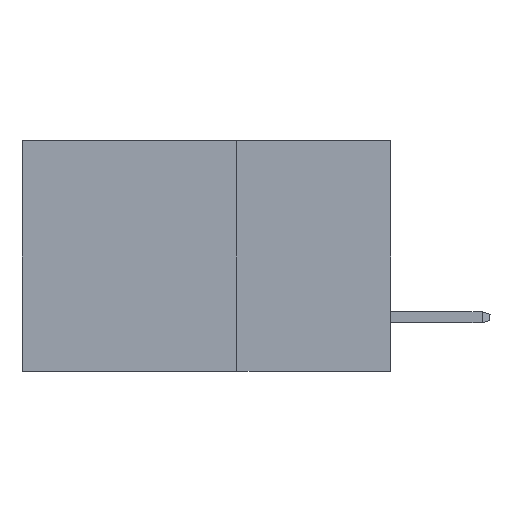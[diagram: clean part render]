
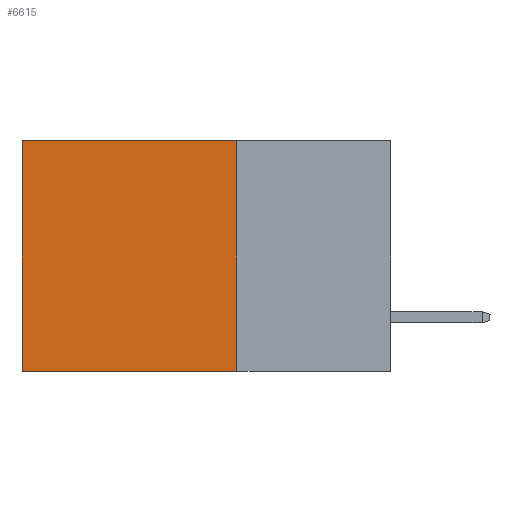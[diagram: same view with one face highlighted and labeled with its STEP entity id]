
A CAD part, left-side view. The second image highlights one B-rep face of the part: STEP entity #6615.
In plain terms, the highlighted planar face has unit normal (-1, 0, 0).
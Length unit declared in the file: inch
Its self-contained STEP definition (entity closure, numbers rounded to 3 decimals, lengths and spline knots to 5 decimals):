
#156 = CARTESIAN_POINT ( 'NONE',  ( 0.2875, 0.25, 0. ) ) ;
#399 = LINE ( 'NONE', #2664, #13032 ) ;
#751 = VERTEX_POINT ( 'NONE', #4200 ) ;
#1082 = LINE ( 'NONE', #13899, #9102 ) ;
#1190 = ORIENTED_EDGE ( 'NONE', *, *, #13895, .F. ) ;
#1422 = EDGE_LOOP ( 'NONE', ( #9313, #1190, #11334, #9749 ) ) ;
#2226 = DIRECTION ( 'NONE',  ( 0., 1., 0. ) ) ;
#2263 = VERTEX_POINT ( 'NONE', #10143 ) ;
#2664 = CARTESIAN_POINT ( 'NONE',  ( 0.2875, 0.25, 0. ) ) ;
#2682 = VECTOR ( 'NONE', #8875, 39.37008 ) ;
#2790 = AXIS2_PLACEMENT_3D ( 'NONE', #8000, #9123, #12720 ) ;
#3269 = LINE ( 'NONE', #14756, #5496 ) ;
#3895 = VERTEX_POINT ( 'NONE', #156 ) ;
#4182 = DIRECTION ( 'NONE',  ( 0., 0., -1. ) ) ;
#4200 = CARTESIAN_POINT ( 'NONE',  ( 0.2875, 0.6, 0. ) ) ;
#5496 = VECTOR ( 'NONE', #4182, 39.37008 ) ;
#6615 = ADVANCED_FACE ( 'NONE', ( #8377 ), #6891, .F. ) ;
#6891 = PLANE ( 'NONE',  #2790 ) ;
#6895 = LINE ( 'NONE', #13558, #2682 ) ;
#8000 = CARTESIAN_POINT ( 'NONE',  ( 0.2875, 0.25, -0.375 ) ) ;
#8339 = EDGE_CURVE ( 'NONE', #3895, #751, #399, .T. ) ;
#8377 = FACE_OUTER_BOUND ( 'NONE', #1422, .T. ) ;
#8875 = DIRECTION ( 'NONE',  ( 0., 0., -1. ) ) ;
#9102 = VECTOR ( 'NONE', #2226, 39.37008 ) ;
#9123 = DIRECTION ( 'NONE',  ( 1., 0., 0. ) ) ;
#9313 = ORIENTED_EDGE ( 'NONE', *, *, #11727, .T. ) ;
#9556 = DIRECTION ( 'NONE',  ( 0., 1., 0. ) ) ;
#9749 = ORIENTED_EDGE ( 'NONE', *, *, #8339, .T. ) ;
#9766 = EDGE_CURVE ( 'NONE', #3895, #2263, #3269, .T. ) ;
#10143 = CARTESIAN_POINT ( 'NONE',  ( 0.2875, 0.25, -0.375 ) ) ;
#11334 = ORIENTED_EDGE ( 'NONE', *, *, #9766, .F. ) ;
#11727 = EDGE_CURVE ( 'NONE', #751, #13119, #6895, .T. ) ;
#12447 = CARTESIAN_POINT ( 'NONE',  ( 0.2875, 0.6, -0.375 ) ) ;
#12720 = DIRECTION ( 'NONE',  ( 0., 0., -1. ) ) ;
#13032 = VECTOR ( 'NONE', #9556, 39.37008 ) ;
#13119 = VERTEX_POINT ( 'NONE', #12447 ) ;
#13558 = CARTESIAN_POINT ( 'NONE',  ( 0.2875, 0.6, -0.375 ) ) ;
#13895 = EDGE_CURVE ( 'NONE', #2263, #13119, #1082, .T. ) ;
#13899 = CARTESIAN_POINT ( 'NONE',  ( 0.2875, 0.25, -0.375 ) ) ;
#14756 = CARTESIAN_POINT ( 'NONE',  ( 0.2875, 0.25, -0.375 ) ) ;
